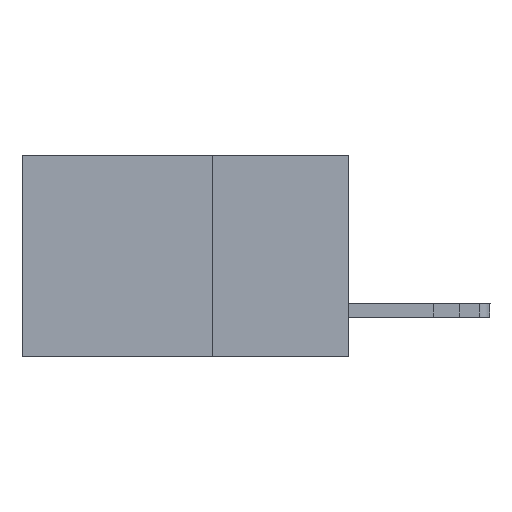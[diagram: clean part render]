
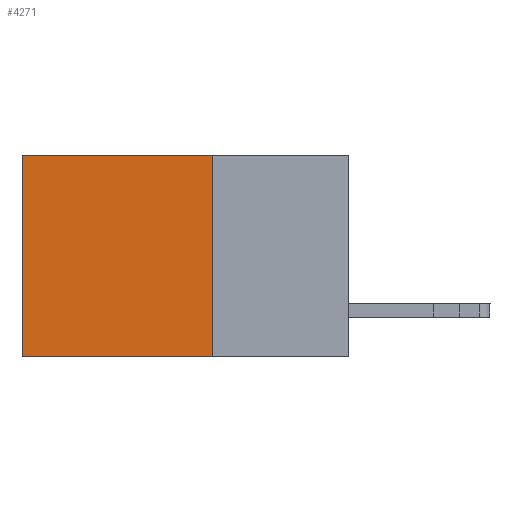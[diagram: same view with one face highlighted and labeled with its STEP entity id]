
A CAD part, left-side view. The second image highlights one B-rep face of the part: STEP entity #4271.
In plain terms, the highlighted planar face has unit normal (-1, 0, 0).
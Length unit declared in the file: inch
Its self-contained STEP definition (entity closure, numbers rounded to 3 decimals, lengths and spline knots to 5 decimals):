
#272 = EDGE_CURVE ( 'NONE', #3108, #12905, #2985, .T. ) ;
#607 = PLANE ( 'NONE',  #10816 ) ;
#1325 = FACE_OUTER_BOUND ( 'NONE', #8296, .T. ) ;
#1592 = ORIENTED_EDGE ( 'NONE', *, *, #10755, .T. ) ;
#1799 = CARTESIAN_POINT ( 'NONE',  ( 0.2615, 0.25, -0.37 ) ) ;
#2432 = ORIENTED_EDGE ( 'NONE', *, *, #272, .T. ) ;
#2768 = VECTOR ( 'NONE', #10921, 39.37008 ) ;
#2985 = LINE ( 'NONE', #7750, #9339 ) ;
#3108 = VERTEX_POINT ( 'NONE', #8199 ) ;
#3278 = LINE ( 'NONE', #11515, #11361 ) ;
#3374 = DIRECTION ( 'NONE',  ( 0., 0., -1. ) ) ;
#3721 = CARTESIAN_POINT ( 'NONE',  ( 0.2615, 0.6, 0. ) ) ;
#4003 = EDGE_CURVE ( 'NONE', #3108, #10723, #6862, .T. ) ;
#4271 = ADVANCED_FACE ( 'NONE', ( #1325 ), #607, .F. ) ;
#5356 = CARTESIAN_POINT ( 'NONE',  ( 0.2615, 0.25, -0.37 ) ) ;
#5416 = DIRECTION ( 'NONE',  ( 1., 0., 0. ) ) ;
#5758 = ORIENTED_EDGE ( 'NONE', *, *, #4003, .F. ) ;
#6781 = CARTESIAN_POINT ( 'NONE',  ( 0.2615, 0.6, -0.37 ) ) ;
#6862 = LINE ( 'NONE', #1799, #2768 ) ;
#6952 = VERTEX_POINT ( 'NONE', #10531 ) ;
#7750 = CARTESIAN_POINT ( 'NONE',  ( 0.2615, 0.25, 0. ) ) ;
#7846 = LINE ( 'NONE', #6781, #10076 ) ;
#7940 = ORIENTED_EDGE ( 'NONE', *, *, #10951, .F. ) ;
#8199 = CARTESIAN_POINT ( 'NONE',  ( 0.2615, 0.25, 0. ) ) ;
#8229 = DIRECTION ( 'NONE',  ( 0., 1., 0. ) ) ;
#8296 = EDGE_LOOP ( 'NONE', ( #1592, #7940, #5758, #2432 ) ) ;
#8709 = CARTESIAN_POINT ( 'NONE',  ( 0.2615, 0.25, -0.37 ) ) ;
#9339 = VECTOR ( 'NONE', #9812, 39.37008 ) ;
#9659 = DIRECTION ( 'NONE',  ( 0., 0., -1. ) ) ;
#9812 = DIRECTION ( 'NONE',  ( 0., 1., 0. ) ) ;
#10076 = VECTOR ( 'NONE', #3374, 39.37008 ) ;
#10531 = CARTESIAN_POINT ( 'NONE',  ( 0.2615, 0.6, -0.37 ) ) ;
#10723 = VERTEX_POINT ( 'NONE', #8709 ) ;
#10755 = EDGE_CURVE ( 'NONE', #12905, #6952, #7846, .T. ) ;
#10816 = AXIS2_PLACEMENT_3D ( 'NONE', #5356, #5416, #9659 ) ;
#10921 = DIRECTION ( 'NONE',  ( 0., 0., -1. ) ) ;
#10951 = EDGE_CURVE ( 'NONE', #10723, #6952, #3278, .T. ) ;
#11361 = VECTOR ( 'NONE', #8229, 39.37008 ) ;
#11515 = CARTESIAN_POINT ( 'NONE',  ( 0.2615, 0.25, -0.37 ) ) ;
#12905 = VERTEX_POINT ( 'NONE', #3721 ) ;
